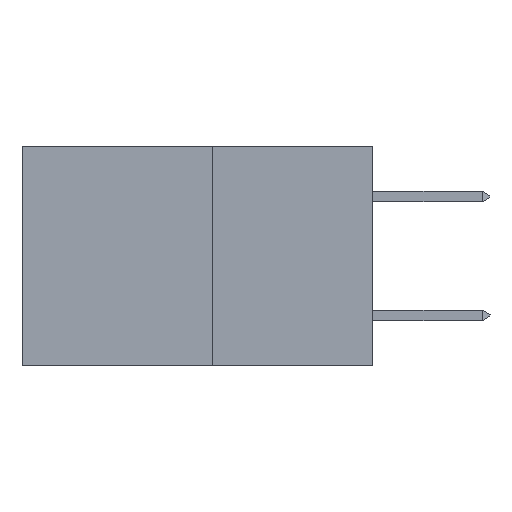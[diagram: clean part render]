
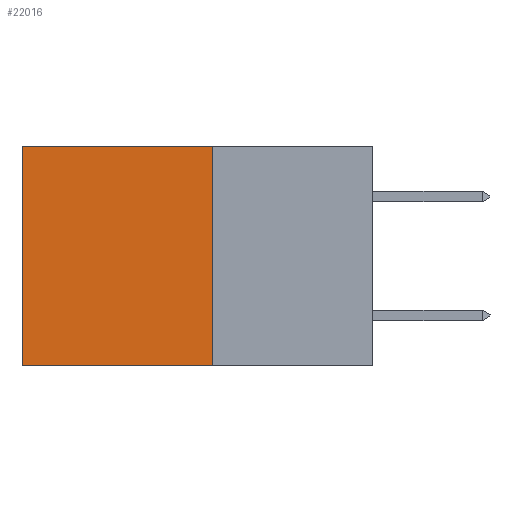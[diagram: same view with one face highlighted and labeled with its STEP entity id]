
A CAD part, left-side view. The second image highlights one B-rep face of the part: STEP entity #22016.
In plain terms, the highlighted planar face has unit normal (-1, 0, 0).
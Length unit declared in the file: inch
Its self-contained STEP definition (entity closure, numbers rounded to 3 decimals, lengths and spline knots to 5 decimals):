
#284 = ORIENTED_EDGE ( 'NONE', *, *, #1616, .F. ) ;
#1615 = VERTEX_POINT ( 'NONE', #15007 ) ;
#1616 = EDGE_CURVE ( 'NONE', #10493, #1615, #13682, .T. ) ;
#2422 = FACE_OUTER_BOUND ( 'NONE', #8924, .T. ) ;
#4150 = EDGE_CURVE ( 'NONE', #18376, #17858, #18526, .T. ) ;
#4249 = VECTOR ( 'NONE', #17027, 39.37008 ) ;
#4315 = VECTOR ( 'NONE', #14459, 39.37008 ) ;
#4650 = VECTOR ( 'NONE', #18520, 39.37008 ) ;
#4915 = CARTESIAN_POINT ( 'NONE',  ( 0.277, 0.27, -0.37 ) ) ;
#5839 = CARTESIAN_POINT ( 'NONE',  ( 0.277, 0.59, 0. ) ) ;
#6317 = LINE ( 'NONE', #7693, #20017 ) ;
#6716 = DIRECTION ( 'NONE',  ( 0., 0., -1. ) ) ;
#7693 = CARTESIAN_POINT ( 'NONE',  ( 0.277, 0.27, 0. ) ) ;
#8924 = EDGE_LOOP ( 'NONE', ( #19838, #21234, #284, #10323 ) ) ;
#9478 = DIRECTION ( 'NONE',  ( 0., 1., 0. ) ) ;
#10323 = ORIENTED_EDGE ( 'NONE', *, *, #10549, .T. ) ;
#10493 = VERTEX_POINT ( 'NONE', #16383 ) ;
#10549 = EDGE_CURVE ( 'NONE', #10493, #18376, #6317, .T. ) ;
#10619 = EDGE_CURVE ( 'NONE', #1615, #17858, #14640, .T. ) ;
#13682 = LINE ( 'NONE', #14982, #4249 ) ;
#14459 = DIRECTION ( 'NONE',  ( 0., 0., -1. ) ) ;
#14494 = CARTESIAN_POINT ( 'NONE',  ( 0.277, 0.59, -0.37 ) ) ;
#14640 = LINE ( 'NONE', #16701, #4650 ) ;
#14982 = CARTESIAN_POINT ( 'NONE',  ( 0.277, 0.27, -0.37 ) ) ;
#15007 = CARTESIAN_POINT ( 'NONE',  ( 0.277, 0.27, -0.37 ) ) ;
#16383 = CARTESIAN_POINT ( 'NONE',  ( 0.277, 0.27, 0. ) ) ;
#16701 = CARTESIAN_POINT ( 'NONE',  ( 0.277, 0.27, -0.37 ) ) ;
#16896 = CARTESIAN_POINT ( 'NONE',  ( 0.277, 0.59, -0.37 ) ) ;
#17027 = DIRECTION ( 'NONE',  ( 0., 0., -1. ) ) ;
#17371 = DIRECTION ( 'NONE',  ( 1., 0., 0. ) ) ;
#17500 = AXIS2_PLACEMENT_3D ( 'NONE', #4915, #17371, #6716 ) ;
#17858 = VERTEX_POINT ( 'NONE', #16896 ) ;
#18376 = VERTEX_POINT ( 'NONE', #5839 ) ;
#18520 = DIRECTION ( 'NONE',  ( 0., 1., 0. ) ) ;
#18526 = LINE ( 'NONE', #14494, #4315 ) ;
#19838 = ORIENTED_EDGE ( 'NONE', *, *, #4150, .T. ) ;
#20017 = VECTOR ( 'NONE', #9478, 39.37008 ) ;
#20916 = PLANE ( 'NONE',  #17500 ) ;
#21234 = ORIENTED_EDGE ( 'NONE', *, *, #10619, .F. ) ;
#22016 = ADVANCED_FACE ( 'NONE', ( #2422 ), #20916, .F. ) ;
